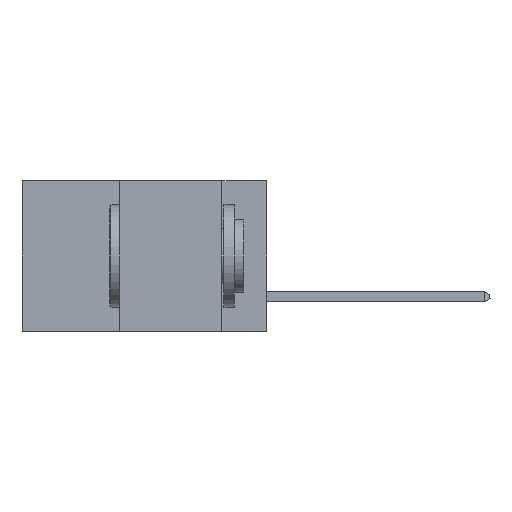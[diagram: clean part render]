
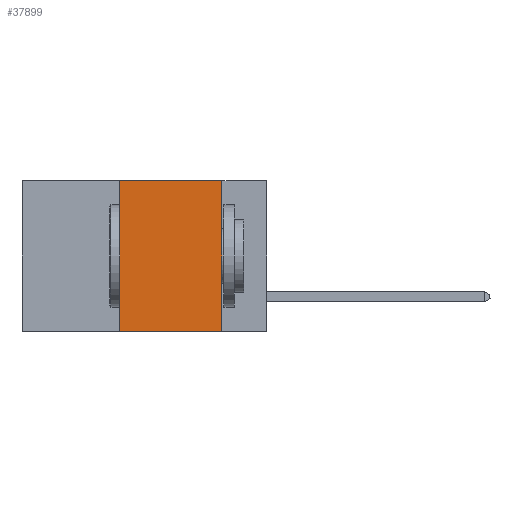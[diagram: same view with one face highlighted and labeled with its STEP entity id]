
A CAD part, left-side view. The second image highlights one B-rep face of the part: STEP entity #37899.
In plain terms, the highlighted planar face has unit normal (-1, 0, 0).
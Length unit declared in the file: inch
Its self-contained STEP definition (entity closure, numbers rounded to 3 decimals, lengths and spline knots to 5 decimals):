
#100 = ORIENTED_EDGE ( 'NONE', *, *, #14579, .F. ) ;
#1874 = CARTESIAN_POINT ( 'NONE',  ( 0., 0.6, -0.37 ) ) ;
#2175 = CARTESIAN_POINT ( 'NONE',  ( 0., 0.11, 0. ) ) ;
#3781 = DIRECTION ( 'NONE',  ( 1., 0., 0. ) ) ;
#4225 = CARTESIAN_POINT ( 'NONE',  ( 0., 0.36, 0. ) ) ;
#6940 = EDGE_CURVE ( 'NONE', #26201, #39676, #12435, .T. ) ;
#7689 = LINE ( 'NONE', #2175, #14416 ) ;
#7772 = ORIENTED_EDGE ( 'NONE', *, *, #15200, .F. ) ;
#8723 = LINE ( 'NONE', #33292, #36158 ) ;
#11276 = FACE_OUTER_BOUND ( 'NONE', #35467, .T. ) ;
#12225 = CARTESIAN_POINT ( 'NONE',  ( 0., 0.11, -0.37 ) ) ;
#12435 = LINE ( 'NONE', #1874, #39368 ) ;
#14416 = VECTOR ( 'NONE', #39125, 39.37008 ) ;
#14579 = EDGE_CURVE ( 'NONE', #26201, #27031, #8723, .T. ) ;
#14712 = LINE ( 'NONE', #35884, #32063 ) ;
#15200 = EDGE_CURVE ( 'NONE', #35782, #39676, #7689, .T. ) ;
#16269 = DIRECTION ( 'NONE',  ( 0., -1., 0. ) ) ;
#21633 = DIRECTION ( 'NONE',  ( 0., 0., 1. ) ) ;
#22145 = CARTESIAN_POINT ( 'NONE',  ( 0., 0.6, 0. ) ) ;
#22279 = PLANE ( 'NONE',  #31521 ) ;
#24977 = DIRECTION ( 'NONE',  ( 0., 0., -1. ) ) ;
#26201 = VERTEX_POINT ( 'NONE', #39283 ) ;
#27031 = VERTEX_POINT ( 'NONE', #4225 ) ;
#28827 = ORIENTED_EDGE ( 'NONE', *, *, #6940, .T. ) ;
#31521 = AXIS2_PLACEMENT_3D ( 'NONE', #22145, #3781, #24977 ) ;
#32063 = VECTOR ( 'NONE', #32798, 39.37008 ) ;
#32798 = DIRECTION ( 'NONE',  ( 0., -1., 0. ) ) ;
#33292 = CARTESIAN_POINT ( 'NONE',  ( 0., 0.36, 0. ) ) ;
#34363 = EDGE_CURVE ( 'NONE', #27031, #35782, #14712, .T. ) ;
#35467 = EDGE_LOOP ( 'NONE', ( #7772, #37791, #100, #28827 ) ) ;
#35782 = VERTEX_POINT ( 'NONE', #37015 ) ;
#35884 = CARTESIAN_POINT ( 'NONE',  ( 0., 0.6, 0. ) ) ;
#36158 = VECTOR ( 'NONE', #21633, 39.37008 ) ;
#37015 = CARTESIAN_POINT ( 'NONE',  ( 0., 0.11, 0. ) ) ;
#37791 = ORIENTED_EDGE ( 'NONE', *, *, #34363, .F. ) ;
#37899 = ADVANCED_FACE ( 'NONE', ( #11276 ), #22279, .F. ) ;
#39125 = DIRECTION ( 'NONE',  ( 0., 0., -1. ) ) ;
#39283 = CARTESIAN_POINT ( 'NONE',  ( 0., 0.36, -0.37 ) ) ;
#39368 = VECTOR ( 'NONE', #16269, 39.37008 ) ;
#39676 = VERTEX_POINT ( 'NONE', #12225 ) ;
